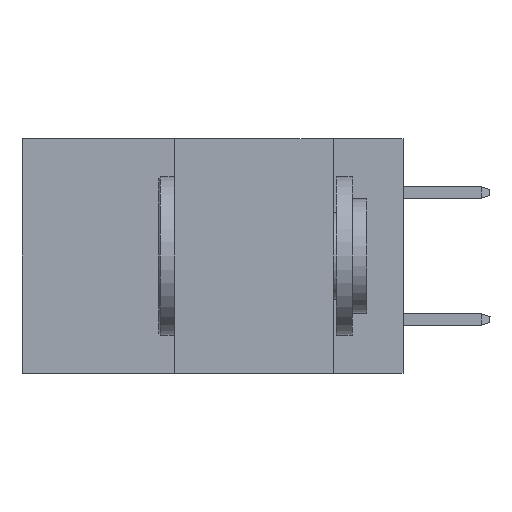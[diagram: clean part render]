
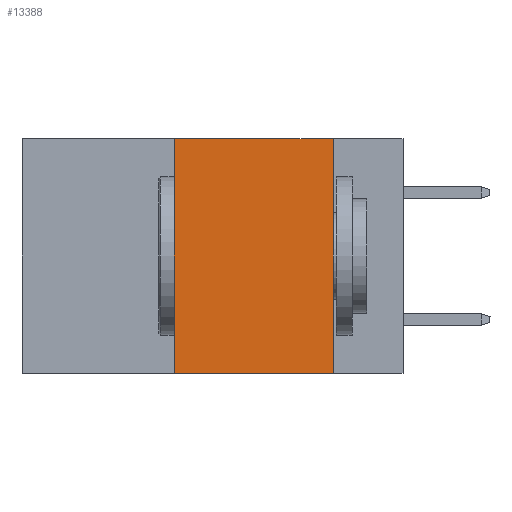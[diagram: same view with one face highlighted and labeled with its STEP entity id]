
A CAD part, left-side view. The second image highlights one B-rep face of the part: STEP entity #13388.
In plain terms, the highlighted planar face has unit normal (-1, 0, 0).
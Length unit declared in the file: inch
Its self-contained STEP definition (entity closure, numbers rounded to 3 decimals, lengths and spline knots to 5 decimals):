
#1850 = CARTESIAN_POINT ( 'NONE',  ( 0., 0.11, 0. ) ) ;
#2034 = VECTOR ( 'NONE', #32373, 39.37008 ) ;
#2237 = LINE ( 'NONE', #1850, #2445 ) ;
#2445 = VECTOR ( 'NONE', #39028, 39.37008 ) ;
#4131 = DIRECTION ( 'NONE',  ( 0., 0., -1. ) ) ;
#4519 = DIRECTION ( 'NONE',  ( 1., 0., 0. ) ) ;
#4915 = CARTESIAN_POINT ( 'NONE',  ( 0., 0.36, -0.37 ) ) ;
#5692 = LINE ( 'NONE', #11946, #15805 ) ;
#6114 = EDGE_CURVE ( 'NONE', #16834, #35705, #21526, .T. ) ;
#7551 = PLANE ( 'NONE',  #21448 ) ;
#10912 = ORIENTED_EDGE ( 'NONE', *, *, #37508, .T. ) ;
#11425 = ORIENTED_EDGE ( 'NONE', *, *, #32709, .F. ) ;
#11946 = CARTESIAN_POINT ( 'NONE',  ( 0., 0.36, 0. ) ) ;
#12504 = CARTESIAN_POINT ( 'NONE',  ( 0., 0.11, -0.37 ) ) ;
#13388 = ADVANCED_FACE ( 'NONE', ( #13797 ), #7551, .F. ) ;
#13704 = CARTESIAN_POINT ( 'NONE',  ( 0., 0.6, -0.37 ) ) ;
#13797 = FACE_OUTER_BOUND ( 'NONE', #21786, .T. ) ;
#13917 = ORIENTED_EDGE ( 'NONE', *, *, #19048, .F. ) ;
#15080 = CARTESIAN_POINT ( 'NONE',  ( 0., 0.6, 0. ) ) ;
#15805 = VECTOR ( 'NONE', #33654, 39.37008 ) ;
#16215 = VERTEX_POINT ( 'NONE', #12504 ) ;
#16834 = VERTEX_POINT ( 'NONE', #34923 ) ;
#19048 = EDGE_CURVE ( 'NONE', #35705, #16215, #2237, .T. ) ;
#19645 = CARTESIAN_POINT ( 'NONE',  ( 0., 0.6, 0. ) ) ;
#21448 = AXIS2_PLACEMENT_3D ( 'NONE', #19645, #4519, #4131 ) ;
#21526 = LINE ( 'NONE', #15080, #35264 ) ;
#21786 = EDGE_LOOP ( 'NONE', ( #13917, #30456, #11425, #10912 ) ) ;
#26173 = VERTEX_POINT ( 'NONE', #4915 ) ;
#29104 = CARTESIAN_POINT ( 'NONE',  ( 0., 0.11, 0. ) ) ;
#30456 = ORIENTED_EDGE ( 'NONE', *, *, #6114, .F. ) ;
#32188 = LINE ( 'NONE', #13704, #2034 ) ;
#32373 = DIRECTION ( 'NONE',  ( 0., -1., 0. ) ) ;
#32709 = EDGE_CURVE ( 'NONE', #26173, #16834, #5692, .T. ) ;
#33654 = DIRECTION ( 'NONE',  ( 0., 0., 1. ) ) ;
#34923 = CARTESIAN_POINT ( 'NONE',  ( 0., 0.36, 0. ) ) ;
#35264 = VECTOR ( 'NONE', #39356, 39.37008 ) ;
#35705 = VERTEX_POINT ( 'NONE', #29104 ) ;
#37508 = EDGE_CURVE ( 'NONE', #26173, #16215, #32188, .T. ) ;
#39028 = DIRECTION ( 'NONE',  ( 0., 0., -1. ) ) ;
#39356 = DIRECTION ( 'NONE',  ( 0., -1., 0. ) ) ;
